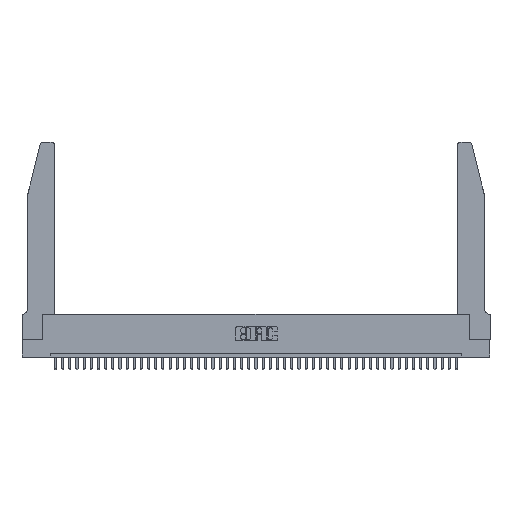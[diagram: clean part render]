
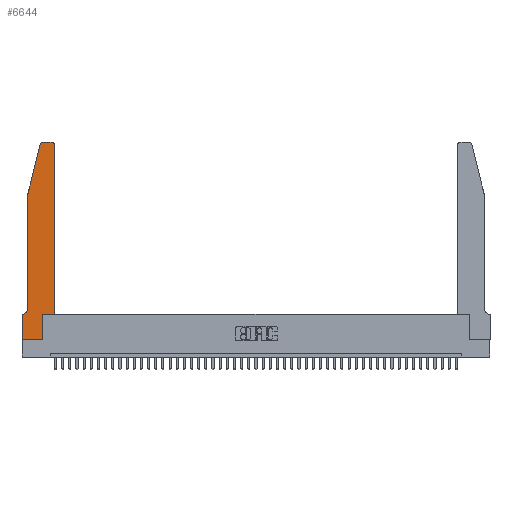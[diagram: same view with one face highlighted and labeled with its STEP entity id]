
A CAD part, top view. The second image highlights one B-rep face of the part: STEP entity #6644.
In plain terms, the highlighted planar face has unit normal (0, 0, 1).
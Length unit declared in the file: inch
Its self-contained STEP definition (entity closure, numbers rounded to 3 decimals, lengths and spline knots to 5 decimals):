
#432 = EDGE_CURVE ( 'NONE', #24773, #29827, #17836, .T. ) ;
#663 = VERTEX_POINT ( 'NONE', #9853 ) ;
#686 = AXIS2_PLACEMENT_3D ( 'NONE', #5051, #15695, #40416 ) ;
#721 = CARTESIAN_POINT ( 'NONE',  ( 0.4205, 2.75, 0.37 ) ) ;
#755 = DIRECTION ( 'NONE',  ( 0., 1., 0. ) ) ;
#1012 = DIRECTION ( 'NONE',  ( -0.239, -0.971, 0. ) ) ;
#1109 = CIRCLE ( 'NONE', #686, 0.03 ) ;
#1165 = ORIENTED_EDGE ( 'NONE', *, *, #25149, .T. ) ;
#1377 = ORIENTED_EDGE ( 'NONE', *, *, #42061, .T. ) ;
#2077 = DIRECTION ( 'NONE',  ( 0., 0., 1. ) ) ;
#2109 = VERTEX_POINT ( 'NONE', #19423 ) ;
#2152 = VERTEX_POINT ( 'NONE', #10302 ) ;
#2503 = VECTOR ( 'NONE', #27573, 39.37008 ) ;
#2795 = CARTESIAN_POINT ( 'NONE',  ( 0.4505, 0.35, 0.37 ) ) ;
#2924 = VECTOR ( 'NONE', #16199, 39.37008 ) ;
#3838 = CARTESIAN_POINT ( 'NONE',  ( 0., 0., 0.37 ) ) ;
#3862 = CARTESIAN_POINT ( 'NONE',  ( 0.0755, 2., 0.37 ) ) ;
#5051 = CARTESIAN_POINT ( 'NONE',  ( 0.4205, 2.72, 0.37 ) ) ;
#5101 = DIRECTION ( 'NONE',  ( 1., 0., 0. ) ) ;
#6644 = ADVANCED_FACE ( 'NONE', ( #7497 ), #30529, .T. ) ;
#7497 = FACE_OUTER_BOUND ( 'NONE', #23591, .T. ) ;
#7960 = CARTESIAN_POINT ( 'NONE',  ( 0.0755, 2., 0.37 ) ) ;
#8654 = CARTESIAN_POINT ( 'NONE',  ( 0., 0., 0.37 ) ) ;
#8707 = VECTOR ( 'NONE', #755, 39.37008 ) ;
#9237 = ORIENTED_EDGE ( 'NONE', *, *, #25768, .T. ) ;
#9412 = EDGE_CURVE ( 'NONE', #35337, #663, #30749, .T. ) ;
#9509 = DIRECTION ( 'NONE',  ( 1., 0., 0. ) ) ;
#9572 = AXIS2_PLACEMENT_3D ( 'NONE', #23624, #17163, #42106 ) ;
#9853 = CARTESIAN_POINT ( 'NONE',  ( 0.0055, 0.35, 0.37 ) ) ;
#10302 = CARTESIAN_POINT ( 'NONE',  ( 0.4505, 2.72, 0.37 ) ) ;
#10331 = DIRECTION ( 'NONE',  ( -1., 0., 0. ) ) ;
#10652 = DIRECTION ( 'NONE',  ( -1., 0., 0. ) ) ;
#11288 = EDGE_CURVE ( 'NONE', #21784, #38136, #30058, .T. ) ;
#11688 = AXIS2_PLACEMENT_3D ( 'NONE', #30688, #2077, #9509 ) ;
#11900 = LINE ( 'NONE', #2795, #2503 ) ;
#12683 = EDGE_CURVE ( 'NONE', #2152, #32008, #1109, .T. ) ;
#13129 = ORIENTED_EDGE ( 'NONE', *, *, #22818, .T. ) ;
#13152 = LINE ( 'NONE', #38964, #8707 ) ;
#13505 = VERTEX_POINT ( 'NONE', #32064 ) ;
#13870 = ORIENTED_EDGE ( 'NONE', *, *, #9412, .T. ) ;
#15695 = DIRECTION ( 'NONE',  ( 0., 0., 1. ) ) ;
#16199 = DIRECTION ( 'NONE',  ( 0., 1., 0. ) ) ;
#16459 = ORIENTED_EDGE ( 'NONE', *, *, #12683, .T. ) ;
#16501 = ORIENTED_EDGE ( 'NONE', *, *, #35768, .T. ) ;
#16947 = VECTOR ( 'NONE', #26017, 39.37008 ) ;
#17163 = DIRECTION ( 'NONE',  ( 0., 0., -1. ) ) ;
#17214 = AXIS2_PLACEMENT_3D ( 'NONE', #19811, #37095, #5101 ) ;
#17813 = LINE ( 'NONE', #24793, #32188 ) ;
#17836 = LINE ( 'NONE', #3838, #28328 ) ;
#17887 = ORIENTED_EDGE ( 'NONE', *, *, #35381, .T. ) ;
#19423 = CARTESIAN_POINT ( 'NONE',  ( 0.284, 2.75, 0.37 ) ) ;
#19811 = CARTESIAN_POINT ( 'NONE',  ( 0.284, 2.72, 0.37 ) ) ;
#20069 = ORIENTED_EDGE ( 'NONE', *, *, #432, .T. ) ;
#21097 = ORIENTED_EDGE ( 'NONE', *, *, #11288, .T. ) ;
#21331 = CARTESIAN_POINT ( 'NONE',  ( 0.4505, 0.35, 0.37 ) ) ;
#21784 = VERTEX_POINT ( 'NONE', #25283 ) ;
#22056 = DIRECTION ( 'NONE',  ( 1., 0., 0. ) ) ;
#22818 = EDGE_CURVE ( 'NONE', #29827, #41699, #13152, .T. ) ;
#23591 = EDGE_LOOP ( 'NONE', ( #1377, #43105, #21097, #38934, #13870, #9237, #16501, #20069, #13129, #17887, #1165, #16459 ) ) ;
#23624 = CARTESIAN_POINT ( 'NONE',  ( 0.0055, 0.42, 0.37 ) ) ;
#23813 = CIRCLE ( 'NONE', #17214, 0.03 ) ;
#23893 = EDGE_CURVE ( 'NONE', #38136, #35337, #26297, .T. ) ;
#24773 = VERTEX_POINT ( 'NONE', #38329 ) ;
#24793 = CARTESIAN_POINT ( 'NONE',  ( 0.0755, 0.35, 0.37 ) ) ;
#25149 = EDGE_CURVE ( 'NONE', #41571, #2152, #30035, .T. ) ;
#25283 = CARTESIAN_POINT ( 'NONE',  ( 0.25487, 2.72718, 0.37 ) ) ;
#25583 = VECTOR ( 'NONE', #40933, 39.37008 ) ;
#25768 = EDGE_CURVE ( 'NONE', #663, #13505, #17813, .T. ) ;
#26017 = DIRECTION ( 'NONE',  ( 0., -1., 0. ) ) ;
#26297 = LINE ( 'NONE', #29770, #16947 ) ;
#27210 = VECTOR ( 'NONE', #10652, 39.37008 ) ;
#27573 = DIRECTION ( 'NONE',  ( 1., 0., 0. ) ) ;
#28328 = VECTOR ( 'NONE', #22056, 39.37008 ) ;
#28370 = VECTOR ( 'NONE', #1012, 39.37008 ) ;
#29770 = CARTESIAN_POINT ( 'NONE',  ( 0.0755, 2., 0.37 ) ) ;
#29827 = VERTEX_POINT ( 'NONE', #38131 ) ;
#29985 = CARTESIAN_POINT ( 'NONE',  ( 0.2865, 0.35, 0.37 ) ) ;
#30035 = LINE ( 'NONE', #43179, #2924 ) ;
#30058 = LINE ( 'NONE', #7960, #28370 ) ;
#30529 = PLANE ( 'NONE',  #11688 ) ;
#30688 = CARTESIAN_POINT ( 'NONE',  ( 0., 0.35, 0.37 ) ) ;
#30749 = CIRCLE ( 'NONE', #9572, 0.07 ) ;
#31287 = CARTESIAN_POINT ( 'NONE',  ( 0.0755, 0.42, 0.37 ) ) ;
#32008 = VERTEX_POINT ( 'NONE', #721 ) ;
#32064 = CARTESIAN_POINT ( 'NONE',  ( 0., 0.35, 0.37 ) ) ;
#32188 = VECTOR ( 'NONE', #10331, 39.37008 ) ;
#32327 = LINE ( 'NONE', #8654, #25583 ) ;
#35337 = VERTEX_POINT ( 'NONE', #31287 ) ;
#35381 = EDGE_CURVE ( 'NONE', #41699, #41571, #11900, .T. ) ;
#35768 = EDGE_CURVE ( 'NONE', #13505, #24773, #32327, .T. ) ;
#35804 = CARTESIAN_POINT ( 'NONE',  ( 0.2605, 2.75, 0.37 ) ) ;
#37095 = DIRECTION ( 'NONE',  ( 0., 0., 1. ) ) ;
#38131 = CARTESIAN_POINT ( 'NONE',  ( 0.2865, 0., 0.37 ) ) ;
#38136 = VERTEX_POINT ( 'NONE', #3862 ) ;
#38329 = CARTESIAN_POINT ( 'NONE',  ( 0., 0., 0.37 ) ) ;
#38438 = EDGE_CURVE ( 'NONE', #2109, #21784, #23813, .T. ) ;
#38934 = ORIENTED_EDGE ( 'NONE', *, *, #23893, .T. ) ;
#38964 = CARTESIAN_POINT ( 'NONE',  ( 0.2865, 0.35, 0.37 ) ) ;
#40416 = DIRECTION ( 'NONE',  ( 1., 0., 0. ) ) ;
#40933 = DIRECTION ( 'NONE',  ( 0., -1., 0. ) ) ;
#41571 = VERTEX_POINT ( 'NONE', #21331 ) ;
#41699 = VERTEX_POINT ( 'NONE', #29985 ) ;
#42061 = EDGE_CURVE ( 'NONE', #32008, #2109, #43163, .T. ) ;
#42106 = DIRECTION ( 'NONE',  ( -1., 0., 0. ) ) ;
#43105 = ORIENTED_EDGE ( 'NONE', *, *, #38438, .T. ) ;
#43163 = LINE ( 'NONE', #35804, #27210 ) ;
#43179 = CARTESIAN_POINT ( 'NONE',  ( 0.4505, 0.35, 0.37 ) ) ;
